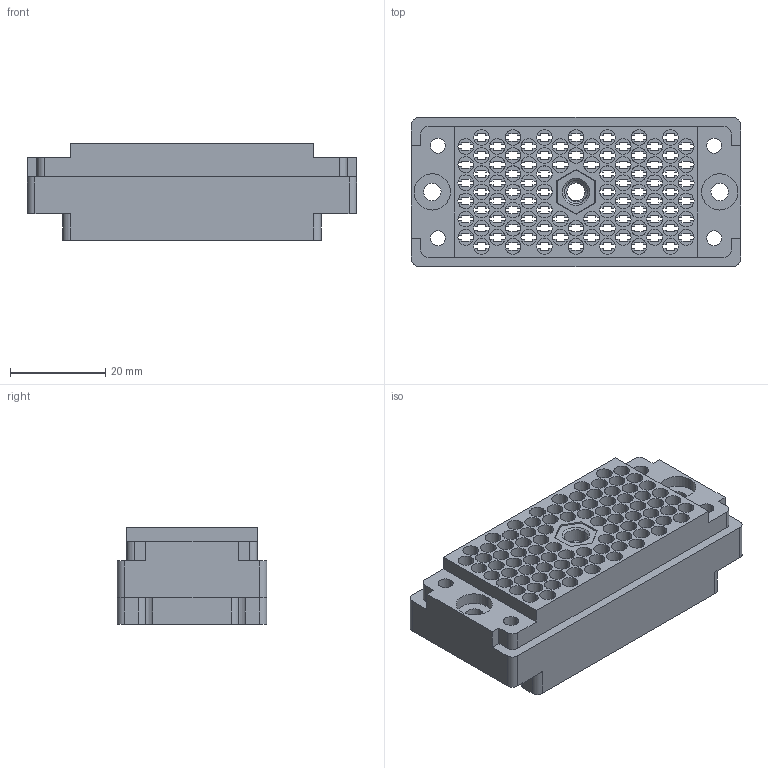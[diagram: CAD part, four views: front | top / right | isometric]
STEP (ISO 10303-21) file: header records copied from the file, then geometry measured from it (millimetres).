
FILE_DESCRIPTION (( 'STEP AP203' ), '1' );
FILE_NAME ('516-090-000-306.STEP', '2020-03-10T15:57:53', ( '' ), ( '' ), 'SwSTEP 2.0', 'SolidWorks 2016', '' );
FILE_SCHEMA (( 'CONFIG_CONTROL_DESIGN' ));
Length unit declared in the file: inch
Products named in the file (3): 516 Plug Insulator_090; 516-252-095-100; 516-090-000-306
Assembly tree (2 placements, depth 2):
  516-090-000-306
    516 Plug Insulator_090
    516-252-095-100
Bounding box: 69.04 x 31.34 x 20.27 mm (x, y, z)
Volume: 16913.2 mm3; surface area: 22659.3 mm2
Topology: 2 solids, 2 shells, 1897 faces, 5625 edges, 3747 vertices
Faces by surface type: plane 1394, cylinder 485, cone 12, bspline 6
Entity records: 65977 total; most frequent: CARTESIAN_POINT 13278, ORIENTED_EDGE 11250, DIRECTION 10698, EDGE_CURVE 5625, VECTOR 4248, LINE 4248, VERTEX_POINT 3747, AXIS2_PLACEMENT_3D 3225
